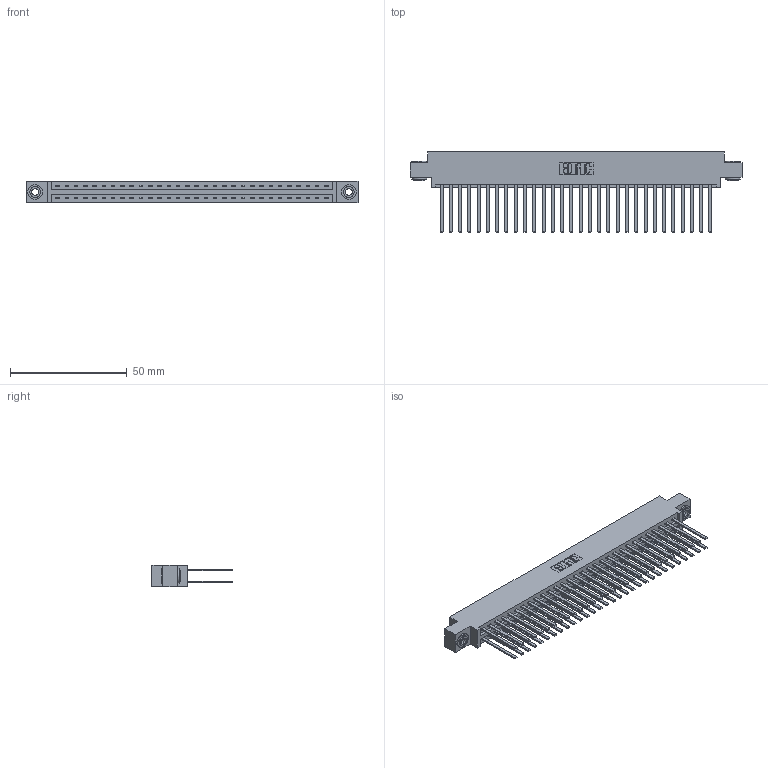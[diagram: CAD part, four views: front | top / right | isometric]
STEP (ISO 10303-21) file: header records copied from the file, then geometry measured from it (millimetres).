
FILE_DESCRIPTION (( 'STEP AP203' ), '1' );
FILE_NAME ('387-060-544-803.STEP', '2019-10-19T13:52:39', ( '' ), ( '' ), 'SwSTEP 2.0', 'SolidWorks 2016', '' );
FILE_SCHEMA (( 'CONFIG_CONTROL_DESIGN' ));
Length unit declared in the file: inch
Products named in the file (4): 337 Part_0.170 Offset - 0.156 Dia-TH; 387-060-544-803; 345-292-001_345-293-144; 345-250-002_345-250-002-102
Assembly tree (63 placements, depth 2):
  387-060-544-803
    337 Part_0.170 Offset - 0.156 Dia-TH
    345-292-001_345-293-144  x60
    345-250-002_345-250-002-102  x2
Bounding box: 141.88 x 34.3 x 9.4 mm (x, y, z)
Volume: 15536.1 mm3; surface area: 20526.9 mm2
Topology: 63 solids, 63 shells, 3036 faces, 8979 edges, 5902 vertices
Faces by surface type: plane 2124, cylinder 904, cone 8
Entity records: 25410 total; most frequent: CARTESIAN_POINT 4265, ORIENTED_EDGE 4194, DIRECTION 3679, EDGE_CURVE 2097, VECTOR 1949, LINE 1949, VERTEX_POINT 1394, AXIS2_PLACEMENT_3D 865
